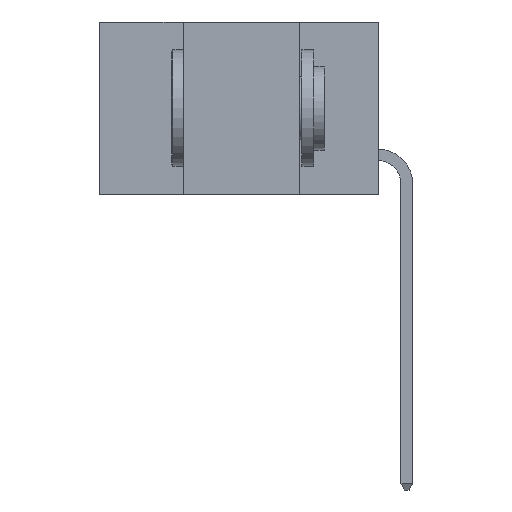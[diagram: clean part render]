
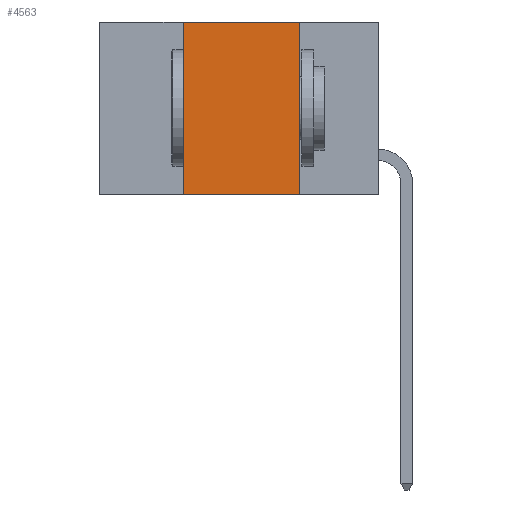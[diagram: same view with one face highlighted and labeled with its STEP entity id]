
A CAD part, left-side view. The second image highlights one B-rep face of the part: STEP entity #4563.
In plain terms, the highlighted planar face has unit normal (-1, 0, 0).
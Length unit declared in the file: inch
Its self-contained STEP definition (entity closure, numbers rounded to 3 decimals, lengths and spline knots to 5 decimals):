
#398 = VERTEX_POINT ( 'NONE', #13077 ) ;
#586 = VERTEX_POINT ( 'NONE', #12064 ) ;
#1459 = CARTESIAN_POINT ( 'NONE',  ( 0., 0.42, -0.37 ) ) ;
#2260 = AXIS2_PLACEMENT_3D ( 'NONE', #11751, #12863, #6167 ) ;
#2288 = EDGE_CURVE ( 'NONE', #7913, #9852, #7470, .T. ) ;
#2420 = CARTESIAN_POINT ( 'NONE',  ( 0., 0.6, 0. ) ) ;
#2484 = ORIENTED_EDGE ( 'NONE', *, *, #12266, .F. ) ;
#2522 = CARTESIAN_POINT ( 'NONE',  ( 0., 0.17, -0.37 ) ) ;
#3411 = ORIENTED_EDGE ( 'NONE', *, *, #5242, .F. ) ;
#3928 = PLANE ( 'NONE',  #2260 ) ;
#4479 = CARTESIAN_POINT ( 'NONE',  ( 0., 0.42, -0.37 ) ) ;
#4563 = ADVANCED_FACE ( 'NONE', ( #5504 ), #3928, .F. ) ;
#4750 = DIRECTION ( 'NONE',  ( 0., 0., -1. ) ) ;
#4847 = LINE ( 'NONE', #2522, #13062 ) ;
#5034 = DIRECTION ( 'NONE',  ( 0., 0., 1. ) ) ;
#5242 = EDGE_CURVE ( 'NONE', #398, #586, #4847, .T. ) ;
#5504 = FACE_OUTER_BOUND ( 'NONE', #12849, .T. ) ;
#5602 = EDGE_CURVE ( 'NONE', #7913, #586, #9936, .T. ) ;
#6167 = DIRECTION ( 'NONE',  ( 0., 0., -1. ) ) ;
#6978 = VECTOR ( 'NONE', #12541, 39.37008 ) ;
#7470 = LINE ( 'NONE', #1459, #10094 ) ;
#7816 = ORIENTED_EDGE ( 'NONE', *, *, #2288, .F. ) ;
#7913 = VERTEX_POINT ( 'NONE', #4479 ) ;
#8071 = CARTESIAN_POINT ( 'NONE',  ( 0., 0.6, -0.37 ) ) ;
#9817 = CARTESIAN_POINT ( 'NONE',  ( 0., 0.42, 0. ) ) ;
#9852 = VERTEX_POINT ( 'NONE', #9817 ) ;
#9936 = LINE ( 'NONE', #8071, #6978 ) ;
#10094 = VECTOR ( 'NONE', #5034, 39.37008 ) ;
#10426 = VECTOR ( 'NONE', #13600, 39.37008 ) ;
#11654 = LINE ( 'NONE', #2420, #10426 ) ;
#11751 = CARTESIAN_POINT ( 'NONE',  ( 0., 0.6, 0. ) ) ;
#12064 = CARTESIAN_POINT ( 'NONE',  ( 0., 0.17, -0.37 ) ) ;
#12266 = EDGE_CURVE ( 'NONE', #9852, #398, #11654, .T. ) ;
#12541 = DIRECTION ( 'NONE',  ( 0., -1., 0. ) ) ;
#12716 = ORIENTED_EDGE ( 'NONE', *, *, #5602, .T. ) ;
#12849 = EDGE_LOOP ( 'NONE', ( #3411, #2484, #7816, #12716 ) ) ;
#12863 = DIRECTION ( 'NONE',  ( 1., 0., 0. ) ) ;
#13062 = VECTOR ( 'NONE', #4750, 39.37008 ) ;
#13077 = CARTESIAN_POINT ( 'NONE',  ( 0., 0.17, 0. ) ) ;
#13600 = DIRECTION ( 'NONE',  ( 0., -1., 0. ) ) ;
